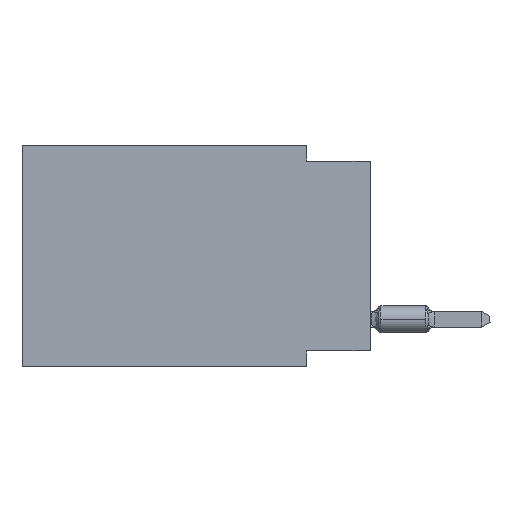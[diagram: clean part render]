
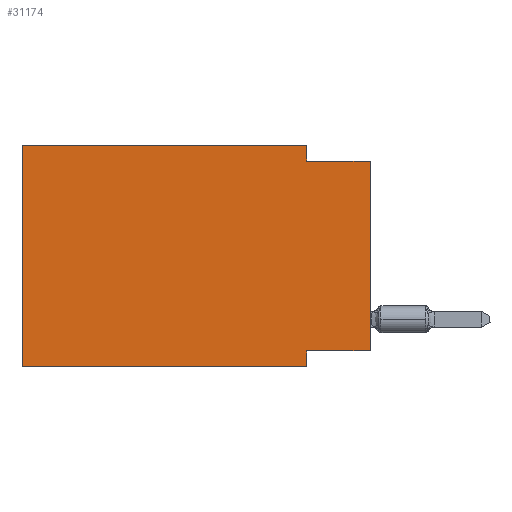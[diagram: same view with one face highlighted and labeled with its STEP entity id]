
A CAD part, left-side view. The second image highlights one B-rep face of the part: STEP entity #31174.
In plain terms, the highlighted planar face has unit normal (-1, 0, 0).
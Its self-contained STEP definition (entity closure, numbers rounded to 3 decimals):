
#600 = CARTESIAN_POINT ( 'NONE',  ( 0., 13.97, 0. ) ) ;
#877 = VERTEX_POINT ( 'NONE', #21576 ) ;
#1296 = ORIENTED_EDGE ( 'NONE', *, *, #5765, .F. ) ;
#1786 = CARTESIAN_POINT ( 'NONE',  ( 0., 2.54, 0. ) ) ;
#1977 = DIRECTION ( 'NONE',  ( 0., 0., -1. ) ) ;
#3208 = DIRECTION ( 'NONE',  ( 0., 0., 1. ) ) ;
#3311 = EDGE_LOOP ( 'NONE', ( #28419, #6506, #9786, #37037, #22132, #27168, #36474, #1296 ) ) ;
#5572 = DIRECTION ( 'NONE',  ( 0., -1., 0. ) ) ;
#5765 = EDGE_CURVE ( 'NONE', #13925, #25849, #32853, .T. ) ;
#6130 = VECTOR ( 'NONE', #39304, 1000. ) ;
#6506 = ORIENTED_EDGE ( 'NONE', *, *, #36809, .F. ) ;
#6835 = CARTESIAN_POINT ( 'NONE',  ( 0., 13.97, 0. ) ) ;
#7363 = VERTEX_POINT ( 'NONE', #22316 ) ;
#7976 = CARTESIAN_POINT ( 'NONE',  ( 0., 0., -8.255 ) ) ;
#9626 = VECTOR ( 'NONE', #24921, 1000. ) ;
#9786 = ORIENTED_EDGE ( 'NONE', *, *, #24630, .F. ) ;
#9853 = DIRECTION ( 'NONE',  ( 1., 0., 0. ) ) ;
#9874 = LINE ( 'NONE', #37379, #9626 ) ;
#9945 = VERTEX_POINT ( 'NONE', #13042 ) ;
#12463 = LINE ( 'NONE', #6835, #30319 ) ;
#13042 = CARTESIAN_POINT ( 'NONE',  ( 0., 2.54, 0. ) ) ;
#13111 = VERTEX_POINT ( 'NONE', #39523 ) ;
#13925 = VERTEX_POINT ( 'NONE', #36007 ) ;
#14342 = VERTEX_POINT ( 'NONE', #20410 ) ;
#14835 = CARTESIAN_POINT ( 'NONE',  ( 0., 13.97, 0. ) ) ;
#15634 = EDGE_CURVE ( 'NONE', #25230, #7363, #29876, .T. ) ;
#17669 = LINE ( 'NONE', #14835, #34780 ) ;
#19179 = VECTOR ( 'NONE', #26226, 1000. ) ;
#19282 = EDGE_CURVE ( 'NONE', #877, #9945, #17669, .T. ) ;
#19766 = EDGE_CURVE ( 'NONE', #25230, #877, #12463, .T. ) ;
#19866 = VECTOR ( 'NONE', #39221, 1000. ) ;
#20410 = CARTESIAN_POINT ( 'NONE',  ( 0., 0., -0.635 ) ) ;
#21576 = CARTESIAN_POINT ( 'NONE',  ( 0., 13.97, 0. ) ) ;
#22132 = ORIENTED_EDGE ( 'NONE', *, *, #19766, .F. ) ;
#22316 = CARTESIAN_POINT ( 'NONE',  ( 0., 2.54, -8.89 ) ) ;
#22728 = CARTESIAN_POINT ( 'NONE',  ( 0., 13.97, -8.89 ) ) ;
#23389 = AXIS2_PLACEMENT_3D ( 'NONE', #600, #9853, #28525 ) ;
#23807 = VECTOR ( 'NONE', #1977, 1000. ) ;
#24630 = EDGE_CURVE ( 'NONE', #9945, #13111, #25884, .T. ) ;
#24631 = CARTESIAN_POINT ( 'NONE',  ( 0., 13.97, -8.89 ) ) ;
#24674 = VECTOR ( 'NONE', #5572, 1000. ) ;
#24921 = DIRECTION ( 'NONE',  ( 0., -1., 0. ) ) ;
#25230 = VERTEX_POINT ( 'NONE', #22728 ) ;
#25849 = VERTEX_POINT ( 'NONE', #39054 ) ;
#25884 = LINE ( 'NONE', #1786, #23807 ) ;
#26226 = DIRECTION ( 'NONE',  ( 0., 1., 0. ) ) ;
#26947 = LINE ( 'NONE', #30739, #19866 ) ;
#27168 = ORIENTED_EDGE ( 'NONE', *, *, #15634, .T. ) ;
#28419 = ORIENTED_EDGE ( 'NONE', *, *, #31761, .T. ) ;
#28525 = DIRECTION ( 'NONE',  ( 0., 0., -1. ) ) ;
#29876 = LINE ( 'NONE', #24631, #24674 ) ;
#30319 = VECTOR ( 'NONE', #3208, 1000. ) ;
#30739 = CARTESIAN_POINT ( 'NONE',  ( 0., 2.54, -8.89 ) ) ;
#31174 = ADVANCED_FACE ( 'NONE', ( #31317 ), #33760, .F. ) ;
#31317 = FACE_OUTER_BOUND ( 'NONE', #3311, .T. ) ;
#31761 = EDGE_CURVE ( 'NONE', #13925, #14342, #38717, .T. ) ;
#32715 = DIRECTION ( 'NONE',  ( 0., -1., 0. ) ) ;
#32853 = LINE ( 'NONE', #7976, #19179 ) ;
#33760 = PLANE ( 'NONE',  #23389 ) ;
#34780 = VECTOR ( 'NONE', #32715, 1000. ) ;
#36007 = CARTESIAN_POINT ( 'NONE',  ( 0., 0., -8.255 ) ) ;
#36474 = ORIENTED_EDGE ( 'NONE', *, *, #36675, .F. ) ;
#36675 = EDGE_CURVE ( 'NONE', #25849, #7363, #26947, .T. ) ;
#36809 = EDGE_CURVE ( 'NONE', #13111, #14342, #9874, .T. ) ;
#37037 = ORIENTED_EDGE ( 'NONE', *, *, #19282, .F. ) ;
#37379 = CARTESIAN_POINT ( 'NONE',  ( 0., 0., -0.635 ) ) ;
#38717 = LINE ( 'NONE', #39105, #6130 ) ;
#39054 = CARTESIAN_POINT ( 'NONE',  ( 0., 2.54, -8.255 ) ) ;
#39105 = CARTESIAN_POINT ( 'NONE',  ( 0., 0., 0. ) ) ;
#39221 = DIRECTION ( 'NONE',  ( 0., 0., -1. ) ) ;
#39304 = DIRECTION ( 'NONE',  ( 0., 0., 1. ) ) ;
#39523 = CARTESIAN_POINT ( 'NONE',  ( 0., 2.54, -0.635 ) ) ;
